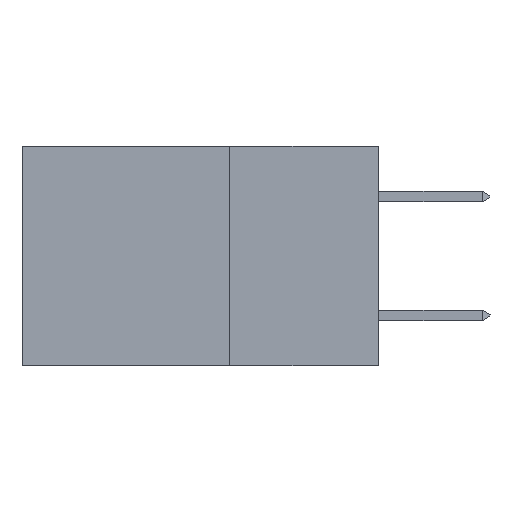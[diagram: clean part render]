
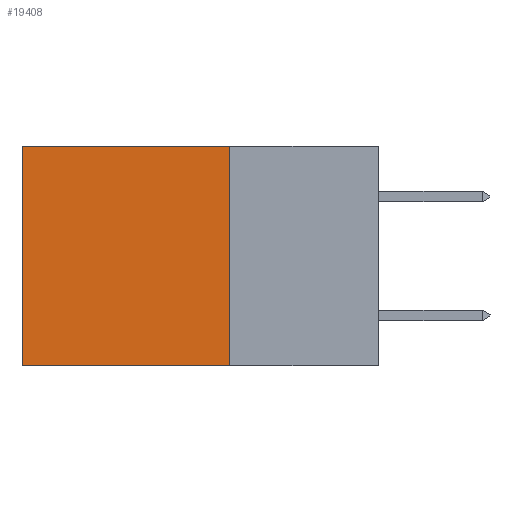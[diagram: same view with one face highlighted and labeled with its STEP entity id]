
A CAD part, left-side view. The second image highlights one B-rep face of the part: STEP entity #19408.
In plain terms, the highlighted planar face has unit normal (-1, 0, 0).
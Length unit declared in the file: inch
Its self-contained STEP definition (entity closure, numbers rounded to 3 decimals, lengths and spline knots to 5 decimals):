
#23 = DIRECTION ( 'NONE',  ( 0., 0., -1. ) ) ;
#106 = LINE ( 'NONE', #18404, #15607 ) ;
#129 = CARTESIAN_POINT ( 'NONE',  ( 0.298, 0.6, 0. ) ) ;
#1885 = VERTEX_POINT ( 'NONE', #16314 ) ;
#2253 = CARTESIAN_POINT ( 'NONE',  ( 0.298, 0.25, 0. ) ) ;
#2796 = DIRECTION ( 'NONE',  ( 0., 0., -1. ) ) ;
#3237 = LINE ( 'NONE', #129, #19686 ) ;
#3434 = DIRECTION ( 'NONE',  ( 0., 1., 0. ) ) ;
#3521 = VECTOR ( 'NONE', #3434, 39.37008 ) ;
#3610 = VERTEX_POINT ( 'NONE', #12112 ) ;
#3620 = EDGE_CURVE ( 'NONE', #8092, #1885, #106, .T. ) ;
#4209 = EDGE_CURVE ( 'NONE', #1885, #3610, #10384, .T. ) ;
#4937 = EDGE_CURVE ( 'NONE', #16439, #3610, #3237, .T. ) ;
#5797 = DIRECTION ( 'NONE',  ( 1., 0., 0. ) ) ;
#6315 = PLANE ( 'NONE',  #13887 ) ;
#8092 = VERTEX_POINT ( 'NONE', #16487 ) ;
#8533 = ORIENTED_EDGE ( 'NONE', *, *, #4209, .F. ) ;
#8547 = ORIENTED_EDGE ( 'NONE', *, *, #4937, .T. ) ;
#10384 = LINE ( 'NONE', #11314, #3521 ) ;
#10899 = ORIENTED_EDGE ( 'NONE', *, *, #3620, .F. ) ;
#11314 = CARTESIAN_POINT ( 'NONE',  ( 0.298, 0.25, -0.37 ) ) ;
#11527 = CARTESIAN_POINT ( 'NONE',  ( 0.298, 0.6, 0. ) ) ;
#11853 = LINE ( 'NONE', #14425, #17728 ) ;
#12043 = DIRECTION ( 'NONE',  ( 0., 0., -1. ) ) ;
#12112 = CARTESIAN_POINT ( 'NONE',  ( 0.298, 0.6, -0.37 ) ) ;
#13504 = EDGE_CURVE ( 'NONE', #8092, #16439, #11853, .T. ) ;
#13850 = FACE_OUTER_BOUND ( 'NONE', #18250, .T. ) ;
#13887 = AXIS2_PLACEMENT_3D ( 'NONE', #2253, #5797, #23 ) ;
#14425 = CARTESIAN_POINT ( 'NONE',  ( 0.298, 0.25, 0. ) ) ;
#15607 = VECTOR ( 'NONE', #12043, 39.37008 ) ;
#16314 = CARTESIAN_POINT ( 'NONE',  ( 0.298, 0.25, -0.37 ) ) ;
#16439 = VERTEX_POINT ( 'NONE', #11527 ) ;
#16487 = CARTESIAN_POINT ( 'NONE',  ( 0.298, 0.25, 0. ) ) ;
#16724 = ORIENTED_EDGE ( 'NONE', *, *, #13504, .T. ) ;
#17728 = VECTOR ( 'NONE', #19172, 39.37008 ) ;
#18250 = EDGE_LOOP ( 'NONE', ( #8547, #8533, #10899, #16724 ) ) ;
#18404 = CARTESIAN_POINT ( 'NONE',  ( 0.298, 0.25, 0. ) ) ;
#19172 = DIRECTION ( 'NONE',  ( 0., 1., 0. ) ) ;
#19408 = ADVANCED_FACE ( 'NONE', ( #13850 ), #6315, .F. ) ;
#19686 = VECTOR ( 'NONE', #2796, 39.37008 ) ;
